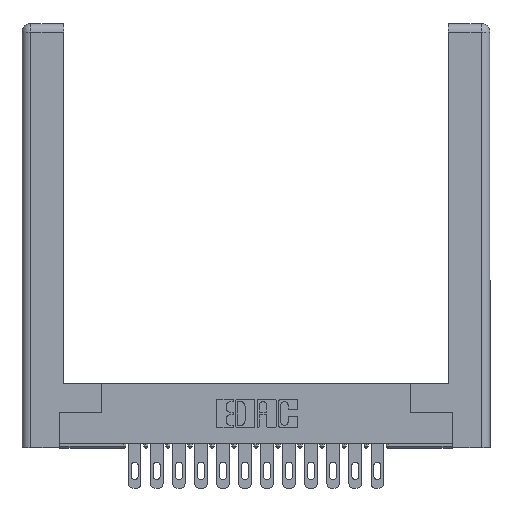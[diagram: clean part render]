
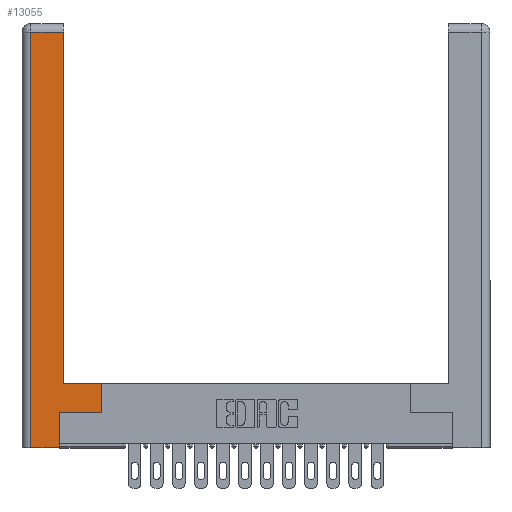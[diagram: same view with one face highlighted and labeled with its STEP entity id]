
A CAD part, top view. The second image highlights one B-rep face of the part: STEP entity #13055.
In plain terms, the highlighted planar face has unit normal (0, 0, 1).
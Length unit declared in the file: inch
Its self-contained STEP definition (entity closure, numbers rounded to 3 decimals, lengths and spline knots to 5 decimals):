
#329 = CARTESIAN_POINT ( 'NONE',  ( 0.295, 0.45, 0. ) ) ;
#861 = EDGE_CURVE ( 'NONE', #3963, #5626, #12489, .T. ) ;
#1073 = DIRECTION ( 'NONE',  ( 0., 0., -1. ) ) ;
#1093 = EDGE_CURVE ( 'NONE', #4558, #5238, #3598, .T. ) ;
#1231 = CARTESIAN_POINT ( 'NONE',  ( 0.0615, 0., 0. ) ) ;
#1450 = EDGE_CURVE ( 'NONE', #13916, #3963, #10088, .T. ) ;
#1771 = DIRECTION ( 'NONE',  ( 0., 1., 0. ) ) ;
#1929 = CARTESIAN_POINT ( 'NONE',  ( 0., 0., 0. ) ) ;
#1952 = ORIENTED_EDGE ( 'NONE', *, *, #861, .T. ) ;
#2033 = VECTOR ( 'NONE', #5211, 39.37008 ) ;
#2034 = DIRECTION ( 'NONE',  ( 0., 1., 0. ) ) ;
#2135 = LINE ( 'NONE', #15884, #17628 ) ;
#3075 = CARTESIAN_POINT ( 'NONE',  ( 0.265, 0.245, 0. ) ) ;
#3598 = LINE ( 'NONE', #1231, #2033 ) ;
#3705 = DIRECTION ( 'NONE',  ( 0., 1., 0. ) ) ;
#3963 = VERTEX_POINT ( 'NONE', #3075 ) ;
#4035 = VERTEX_POINT ( 'NONE', #5047 ) ;
#4171 = CARTESIAN_POINT ( 'NONE',  ( 0.565, 0.245, 0. ) ) ;
#4385 = CARTESIAN_POINT ( 'NONE',  ( 0.295, 2.94, 0. ) ) ;
#4558 = VERTEX_POINT ( 'NONE', #12897 ) ;
#4583 = LINE ( 'NONE', #329, #16894 ) ;
#5047 = CARTESIAN_POINT ( 'NONE',  ( 0.295, 0.45, 0. ) ) ;
#5142 = DIRECTION ( 'NONE',  ( -1., 0., 0. ) ) ;
#5211 = DIRECTION ( 'NONE',  ( 0., -1., 0. ) ) ;
#5238 = VERTEX_POINT ( 'NONE', #17556 ) ;
#5626 = VERTEX_POINT ( 'NONE', #14808 ) ;
#5794 = EDGE_CURVE ( 'NONE', #13545, #4035, #4583, .T. ) ;
#5990 = DIRECTION ( 'NONE',  ( 1., 0., 0. ) ) ;
#7365 = VECTOR ( 'NONE', #2034, 39.37008 ) ;
#7668 = ORIENTED_EDGE ( 'NONE', *, *, #1450, .T. ) ;
#8650 = CARTESIAN_POINT ( 'NONE',  ( 0.265, 0.245, 0. ) ) ;
#8997 = LINE ( 'NONE', #11793, #7365 ) ;
#9003 = VECTOR ( 'NONE', #15207, 39.37008 ) ;
#9403 = EDGE_CURVE ( 'NONE', #5238, #13916, #12322, .T. ) ;
#10088 = LINE ( 'NONE', #8650, #13513 ) ;
#10426 = EDGE_CURVE ( 'NONE', #13759, #4558, #2135, .T. ) ;
#10498 = ORIENTED_EDGE ( 'NONE', *, *, #16709, .T. ) ;
#11231 = EDGE_LOOP ( 'NONE', ( #10498, #13030, #17577, #14080, #7668, #1952, #16209, #13223 ) ) ;
#11235 = VECTOR ( 'NONE', #5990, 39.37008 ) ;
#11679 = CARTESIAN_POINT ( 'NONE',  ( 0.265, 0., 0. ) ) ;
#11793 = CARTESIAN_POINT ( 'NONE',  ( 0.565, 0.45, 0. ) ) ;
#11921 = FACE_OUTER_BOUND ( 'NONE', #11231, .T. ) ;
#11928 = CARTESIAN_POINT ( 'NONE',  ( 0.295, 3., 0. ) ) ;
#12322 = LINE ( 'NONE', #11679, #11235 ) ;
#12489 = LINE ( 'NONE', #4171, #9003 ) ;
#12897 = CARTESIAN_POINT ( 'NONE',  ( 0.0615, 2.94, 0. ) ) ;
#12952 = PLANE ( 'NONE',  #17706 ) ;
#13030 = ORIENTED_EDGE ( 'NONE', *, *, #10426, .T. ) ;
#13055 = ADVANCED_FACE ( 'NONE', ( #11921 ), #12952, .F. ) ;
#13223 = ORIENTED_EDGE ( 'NONE', *, *, #5794, .T. ) ;
#13287 = LINE ( 'NONE', #11928, #14039 ) ;
#13513 = VECTOR ( 'NONE', #1771, 39.37008 ) ;
#13545 = VERTEX_POINT ( 'NONE', #17521 ) ;
#13759 = VERTEX_POINT ( 'NONE', #4385 ) ;
#13916 = VERTEX_POINT ( 'NONE', #14685 ) ;
#14039 = VECTOR ( 'NONE', #3705, 39.37008 ) ;
#14080 = ORIENTED_EDGE ( 'NONE', *, *, #9403, .T. ) ;
#14685 = CARTESIAN_POINT ( 'NONE',  ( 0.265, 0., 0. ) ) ;
#14808 = CARTESIAN_POINT ( 'NONE',  ( 0.565, 0.245, 0. ) ) ;
#15186 = EDGE_CURVE ( 'NONE', #5626, #13545, #8997, .T. ) ;
#15207 = DIRECTION ( 'NONE',  ( 1., 0., 0. ) ) ;
#15707 = DIRECTION ( 'NONE',  ( -1., 0., 0. ) ) ;
#15884 = CARTESIAN_POINT ( 'NONE',  ( 0.0615, 2.94, 0. ) ) ;
#16209 = ORIENTED_EDGE ( 'NONE', *, *, #15186, .T. ) ;
#16709 = EDGE_CURVE ( 'NONE', #4035, #13759, #13287, .T. ) ;
#16894 = VECTOR ( 'NONE', #15707, 39.37008 ) ;
#17515 = DIRECTION ( 'NONE',  ( -1., 0., 0. ) ) ;
#17521 = CARTESIAN_POINT ( 'NONE',  ( 0.565, 0.45, 0. ) ) ;
#17556 = CARTESIAN_POINT ( 'NONE',  ( 0.0615, 0., 0. ) ) ;
#17577 = ORIENTED_EDGE ( 'NONE', *, *, #1093, .T. ) ;
#17628 = VECTOR ( 'NONE', #17515, 39.37008 ) ;
#17706 = AXIS2_PLACEMENT_3D ( 'NONE', #1929, #1073, #5142 ) ;
